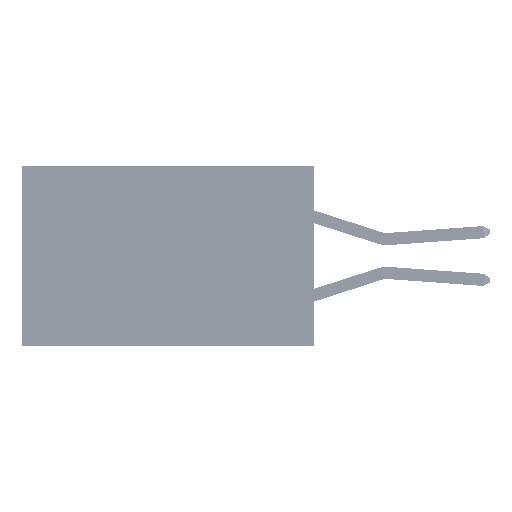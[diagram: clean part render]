
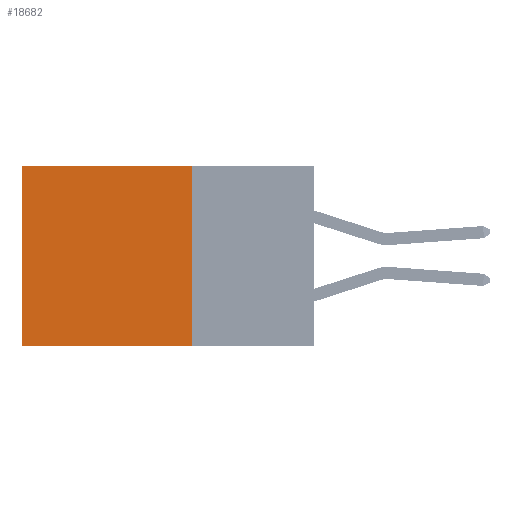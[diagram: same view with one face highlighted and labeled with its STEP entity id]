
A CAD part, left-side view. The second image highlights one B-rep face of the part: STEP entity #18682.
In plain terms, the highlighted planar face has unit normal (-1, 0, 0).
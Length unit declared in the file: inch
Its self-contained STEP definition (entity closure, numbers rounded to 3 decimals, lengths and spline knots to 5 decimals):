
#7 = CARTESIAN_POINT ( 'NONE',  ( 0.2875, 0.25, 0. ) ) ;
#1218 = VECTOR ( 'NONE', #26109, 39.37008 ) ;
#1647 = LINE ( 'NONE', #5354, #42681 ) ;
#2505 = LINE ( 'NONE', #21980, #1218 ) ;
#4409 = CARTESIAN_POINT ( 'NONE',  ( 0.2875, 0.25, 0. ) ) ;
#5354 = CARTESIAN_POINT ( 'NONE',  ( 0.2875, 0.6, 0. ) ) ;
#5973 = EDGE_LOOP ( 'NONE', ( #43374, #45463, #12484, #20361 ) ) ;
#6270 = LINE ( 'NONE', #7, #10641 ) ;
#9785 = CARTESIAN_POINT ( 'NONE',  ( 0.2875, 0.25, 0. ) ) ;
#10641 = VECTOR ( 'NONE', #41024, 39.37008 ) ;
#10777 = VECTOR ( 'NONE', #30410, 39.37008 ) ;
#11460 = VERTEX_POINT ( 'NONE', #4409 ) ;
#12484 = ORIENTED_EDGE ( 'NONE', *, *, #23295, .F. ) ;
#13521 = EDGE_CURVE ( 'NONE', #21194, #34921, #1647, .T. ) ;
#18682 = ADVANCED_FACE ( 'NONE', ( #22954 ), #22733, .F. ) ;
#20361 = ORIENTED_EDGE ( 'NONE', *, *, #46005, .T. ) ;
#21194 = VERTEX_POINT ( 'NONE', #48842 ) ;
#21443 = DIRECTION ( 'NONE',  ( 0., 0., -1. ) ) ;
#21980 = CARTESIAN_POINT ( 'NONE',  ( 0.2875, 0.25, -0.37 ) ) ;
#22733 = PLANE ( 'NONE',  #43393 ) ;
#22916 = CARTESIAN_POINT ( 'NONE',  ( 0.2875, 0.25, 0. ) ) ;
#22954 = FACE_OUTER_BOUND ( 'NONE', #5973, .T. ) ;
#23295 = EDGE_CURVE ( 'NONE', #11460, #38086, #31987, .T. ) ;
#26109 = DIRECTION ( 'NONE',  ( 0., 1., 0. ) ) ;
#26678 = DIRECTION ( 'NONE',  ( 1., 0., 0. ) ) ;
#27004 = CARTESIAN_POINT ( 'NONE',  ( 0.2875, 0.6, -0.37 ) ) ;
#30410 = DIRECTION ( 'NONE',  ( 0., 0., -1. ) ) ;
#31987 = LINE ( 'NONE', #9785, #10777 ) ;
#33558 = EDGE_CURVE ( 'NONE', #38086, #34921, #2505, .T. ) ;
#33615 = CARTESIAN_POINT ( 'NONE',  ( 0.2875, 0.25, -0.37 ) ) ;
#34921 = VERTEX_POINT ( 'NONE', #27004 ) ;
#38086 = VERTEX_POINT ( 'NONE', #33615 ) ;
#41024 = DIRECTION ( 'NONE',  ( 0., 1., 0. ) ) ;
#42681 = VECTOR ( 'NONE', #21443, 39.37008 ) ;
#43374 = ORIENTED_EDGE ( 'NONE', *, *, #13521, .T. ) ;
#43393 = AXIS2_PLACEMENT_3D ( 'NONE', #22916, #26678, #47157 ) ;
#45463 = ORIENTED_EDGE ( 'NONE', *, *, #33558, .F. ) ;
#46005 = EDGE_CURVE ( 'NONE', #11460, #21194, #6270, .T. ) ;
#47157 = DIRECTION ( 'NONE',  ( 0., 0., -1. ) ) ;
#48842 = CARTESIAN_POINT ( 'NONE',  ( 0.2875, 0.6, 0. ) ) ;
